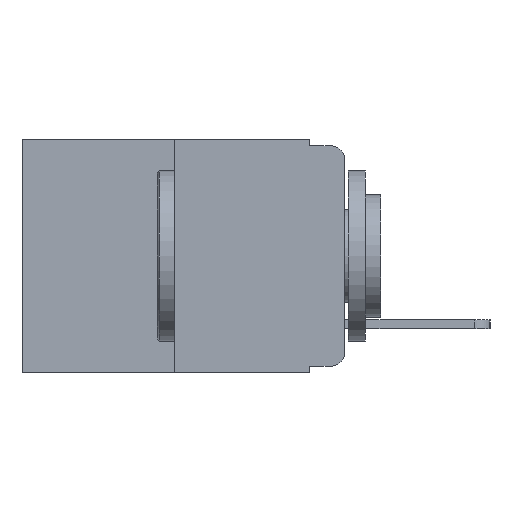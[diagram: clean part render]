
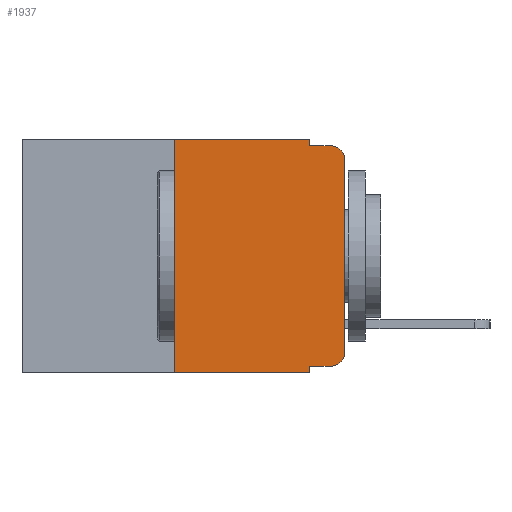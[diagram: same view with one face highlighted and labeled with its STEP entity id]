
A CAD part, left-side view. The second image highlights one B-rep face of the part: STEP entity #1937.
In plain terms, the highlighted planar face has unit normal (-1, 0, 0).
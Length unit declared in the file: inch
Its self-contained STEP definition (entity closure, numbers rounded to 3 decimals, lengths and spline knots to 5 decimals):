
#594 = CARTESIAN_POINT ( 'NONE',  ( 0., 0., -0.03 ) ) ;
#643 = FACE_OUTER_BOUND ( 'NONE', #2911, .T. ) ;
#751 = CARTESIAN_POINT ( 'NONE',  ( 0., 0.051, 0. ) ) ;
#864 = CARTESIAN_POINT ( 'NONE',  ( 0., 0.051, -0.333 ) ) ;
#1059 = PLANE ( 'NONE',  #7220 ) ;
#1793 = ORIENTED_EDGE ( 'NONE', *, *, #7053, .T. ) ;
#1937 = ADVANCED_FACE ( 'NONE', ( #643 ), #1059, .F. ) ;
#2005 = VECTOR ( 'NONE', #2063, 39.37008 ) ;
#2017 = ORIENTED_EDGE ( 'NONE', *, *, #7054, .F. ) ;
#2063 = DIRECTION ( 'NONE',  ( 0., 0., 1. ) ) ;
#2280 = ORIENTED_EDGE ( 'NONE', *, *, #7063, .F. ) ;
#2350 = VECTOR ( 'NONE', #3043, 39.37008 ) ;
#2547 = CARTESIAN_POINT ( 'NONE',  ( 0., 0.473, -0.343 ) ) ;
#2564 = VECTOR ( 'NONE', #7243, 39.37008 ) ;
#2597 = ORIENTED_EDGE ( 'NONE', *, *, #5650, .F. ) ;
#2695 = CIRCLE ( 'NONE', #10891, 0.02 ) ;
#2890 = DIRECTION ( 'NONE',  ( 0., 0., -1. ) ) ;
#2911 = EDGE_LOOP ( 'NONE', ( #7106, #1793, #2017, #2280, #2597, #2924, #2950, #3032, #3063, #3279 ) ) ;
#2924 = ORIENTED_EDGE ( 'NONE', *, *, #7083, .F. ) ;
#2950 = ORIENTED_EDGE ( 'NONE', *, *, #6549, .T. ) ;
#3004 = CARTESIAN_POINT ( 'NONE',  ( 0., 0.25, -0.343 ) ) ;
#3032 = ORIENTED_EDGE ( 'NONE', *, *, #7084, .F. ) ;
#3043 = DIRECTION ( 'NONE',  ( 0., -1., 0. ) ) ;
#3063 = ORIENTED_EDGE ( 'NONE', *, *, #7097, .T. ) ;
#3089 = CARTESIAN_POINT ( 'NONE',  ( 0., 0.02, -0.03 ) ) ;
#3279 = ORIENTED_EDGE ( 'NONE', *, *, #7122, .T. ) ;
#3415 = CARTESIAN_POINT ( 'NONE',  ( 0., 0.473, 0. ) ) ;
#4024 = CARTESIAN_POINT ( 'NONE',  ( 0., 0., 0. ) ) ;
#4028 = CARTESIAN_POINT ( 'NONE',  ( 0., 0.051, 0. ) ) ;
#4103 = DIRECTION ( 'NONE',  ( 0., 0., -1. ) ) ;
#4194 = DIRECTION ( 'NONE',  ( -1., 0., 0. ) ) ;
#4453 = LINE ( 'NONE', #864, #11593 ) ;
#4778 = LINE ( 'NONE', #6055, #7258 ) ;
#5074 = LINE ( 'NONE', #751, #9647 ) ;
#5315 = DIRECTION ( 'NONE',  ( 1., 0., 0. ) ) ;
#5324 = VERTEX_POINT ( 'NONE', #6899 ) ;
#5650 = EDGE_CURVE ( 'NONE', #9957, #9680, #12283, .T. ) ;
#6026 = DIRECTION ( 'NONE',  ( 0., 0., 1. ) ) ;
#6055 = CARTESIAN_POINT ( 'NONE',  ( 0., 0.051, 0. ) ) ;
#6127 = CARTESIAN_POINT ( 'NONE',  ( 0., 0., -0.313 ) ) ;
#6378 = VERTEX_POINT ( 'NONE', #6127 ) ;
#6549 = EDGE_CURVE ( 'NONE', #9689, #8295, #7268, .T. ) ;
#6899 = CARTESIAN_POINT ( 'NONE',  ( 0., 0.02, -0.01 ) ) ;
#6925 = VERTEX_POINT ( 'NONE', #7788 ) ;
#6992 = CARTESIAN_POINT ( 'NONE',  ( 0., 0.25, 0. ) ) ;
#7019 = EDGE_CURVE ( 'NONE', #6378, #11252, #9910, .T. ) ;
#7053 = EDGE_CURVE ( 'NONE', #11252, #5324, #2695, .T. ) ;
#7054 = EDGE_CURVE ( 'NONE', #9200, #5324, #7823, .T. ) ;
#7063 = EDGE_CURVE ( 'NONE', #9680, #9200, #5074, .T. ) ;
#7083 = EDGE_CURVE ( 'NONE', #9689, #9957, #11864, .T. ) ;
#7084 = EDGE_CURVE ( 'NONE', #11654, #8295, #4778, .T. ) ;
#7097 = EDGE_CURVE ( 'NONE', #11654, #6925, #4453, .T. ) ;
#7106 = ORIENTED_EDGE ( 'NONE', *, *, #7019, .T. ) ;
#7122 = EDGE_CURVE ( 'NONE', #6925, #6378, #9377, .T. ) ;
#7220 = AXIS2_PLACEMENT_3D ( 'NONE', #9374, #5315, #2890 ) ;
#7243 = DIRECTION ( 'NONE',  ( 0., -1., 0. ) ) ;
#7258 = VECTOR ( 'NONE', #9706, 39.37008 ) ;
#7268 = LINE ( 'NONE', #2547, #7542 ) ;
#7528 = VECTOR ( 'NONE', #6026, 39.37008 ) ;
#7542 = VECTOR ( 'NONE', #10068, 39.37008 ) ;
#7788 = CARTESIAN_POINT ( 'NONE',  ( 0., 0.02, -0.333 ) ) ;
#7823 = LINE ( 'NONE', #7866, #2350 ) ;
#7866 = CARTESIAN_POINT ( 'NONE',  ( 0., 0.051, -0.01 ) ) ;
#7930 = DIRECTION ( 'NONE',  ( 0., -1., 0. ) ) ;
#8295 = VERTEX_POINT ( 'NONE', #8859 ) ;
#8786 = DIRECTION ( 'NONE',  ( 0., 0., -1. ) ) ;
#8859 = CARTESIAN_POINT ( 'NONE',  ( 0., 0.051, -0.343 ) ) ;
#9200 = VERTEX_POINT ( 'NONE', #12329 ) ;
#9374 = CARTESIAN_POINT ( 'NONE',  ( 0., 0.473, 0. ) ) ;
#9377 = CIRCLE ( 'NONE', #10344, 0.02 ) ;
#9647 = VECTOR ( 'NONE', #8786, 39.37008 ) ;
#9668 = DIRECTION ( 'NONE',  ( -1., 0., 0. ) ) ;
#9680 = VERTEX_POINT ( 'NONE', #4028 ) ;
#9689 = VERTEX_POINT ( 'NONE', #3004 ) ;
#9706 = DIRECTION ( 'NONE',  ( 0., 0., -1. ) ) ;
#9734 = CARTESIAN_POINT ( 'NONE',  ( 0., 0.02, -0.313 ) ) ;
#9910 = LINE ( 'NONE', #4024, #7528 ) ;
#9957 = VERTEX_POINT ( 'NONE', #10982 ) ;
#10068 = DIRECTION ( 'NONE',  ( 0., -1., 0. ) ) ;
#10344 = AXIS2_PLACEMENT_3D ( 'NONE', #9734, #4194, #10545 ) ;
#10545 = DIRECTION ( 'NONE',  ( 0., 0., -1. ) ) ;
#10891 = AXIS2_PLACEMENT_3D ( 'NONE', #3089, #9668, #4103 ) ;
#10982 = CARTESIAN_POINT ( 'NONE',  ( 0., 0.25, 0. ) ) ;
#11252 = VERTEX_POINT ( 'NONE', #594 ) ;
#11593 = VECTOR ( 'NONE', #7930, 39.37008 ) ;
#11654 = VERTEX_POINT ( 'NONE', #11686 ) ;
#11686 = CARTESIAN_POINT ( 'NONE',  ( 0., 0.051, -0.333 ) ) ;
#11864 = LINE ( 'NONE', #6992, #2005 ) ;
#12283 = LINE ( 'NONE', #3415, #2564 ) ;
#12329 = CARTESIAN_POINT ( 'NONE',  ( 0., 0.051, -0.01 ) ) ;
